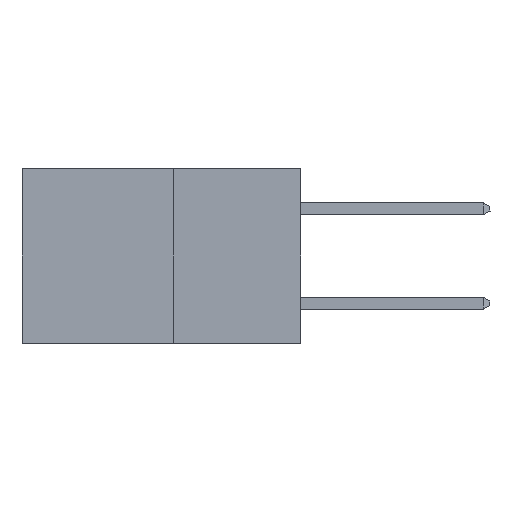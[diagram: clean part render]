
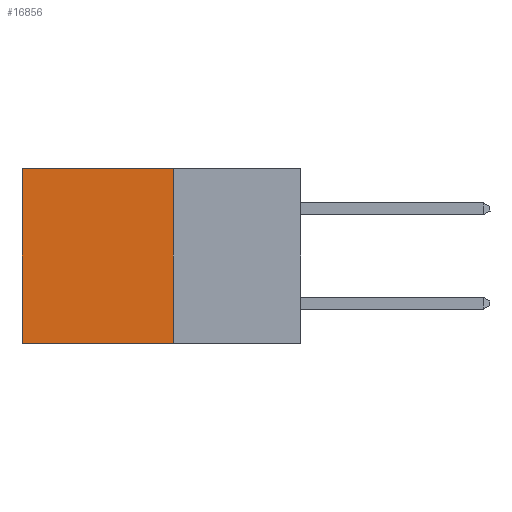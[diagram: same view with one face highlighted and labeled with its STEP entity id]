
A CAD part, left-side view. The second image highlights one B-rep face of the part: STEP entity #16856.
In plain terms, the highlighted planar face has unit normal (-1, 0, 0).
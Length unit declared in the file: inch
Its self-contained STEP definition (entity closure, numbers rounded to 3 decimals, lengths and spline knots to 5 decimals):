
#135 = DIRECTION ( 'NONE',  ( 1., 0., 0. ) ) ;
#337 = DIRECTION ( 'NONE',  ( 0., 0., -1. ) ) ;
#3577 = ORIENTED_EDGE ( 'NONE', *, *, #6771, .T. ) ;
#4001 = VECTOR ( 'NONE', #11447, 39.37008 ) ;
#5173 = CARTESIAN_POINT ( 'NONE',  ( 0.277, 0.59, -0.37 ) ) ;
#6661 = PLANE ( 'NONE',  #17743 ) ;
#6771 = EDGE_CURVE ( 'NONE', #9305, #20219, #13177, .T. ) ;
#7927 = EDGE_LOOP ( 'NONE', ( #3577, #9611, #12862, #16972 ) ) ;
#8671 = VECTOR ( 'NONE', #20311, 39.37008 ) ;
#9046 = VECTOR ( 'NONE', #18298, 39.37008 ) ;
#9305 = VERTEX_POINT ( 'NONE', #15553 ) ;
#9477 = CARTESIAN_POINT ( 'NONE',  ( 0.277, 0.27, 0. ) ) ;
#9611 = ORIENTED_EDGE ( 'NONE', *, *, #10947, .F. ) ;
#9889 = CARTESIAN_POINT ( 'NONE',  ( 0.277, 0.27, -0.37 ) ) ;
#10947 = EDGE_CURVE ( 'NONE', #12393, #20219, #12300, .T. ) ;
#11379 = EDGE_CURVE ( 'NONE', #12591, #9305, #17414, .T. ) ;
#11447 = DIRECTION ( 'NONE',  ( 0., 1., 0. ) ) ;
#12040 = CARTESIAN_POINT ( 'NONE',  ( 0.277, 0.59, -0.37 ) ) ;
#12300 = LINE ( 'NONE', #9889, #4001 ) ;
#12393 = VERTEX_POINT ( 'NONE', #12434 ) ;
#12434 = CARTESIAN_POINT ( 'NONE',  ( 0.277, 0.27, -0.37 ) ) ;
#12591 = VERTEX_POINT ( 'NONE', #12832 ) ;
#12832 = CARTESIAN_POINT ( 'NONE',  ( 0.277, 0.27, 0. ) ) ;
#12862 = ORIENTED_EDGE ( 'NONE', *, *, #15472, .F. ) ;
#13177 = LINE ( 'NONE', #12040, #9046 ) ;
#14439 = CARTESIAN_POINT ( 'NONE',  ( 0.277, 0.27, -0.37 ) ) ;
#14597 = VECTOR ( 'NONE', #337, 39.37008 ) ;
#15472 = EDGE_CURVE ( 'NONE', #12591, #12393, #18253, .T. ) ;
#15553 = CARTESIAN_POINT ( 'NONE',  ( 0.277, 0.59, 0. ) ) ;
#16856 = ADVANCED_FACE ( 'NONE', ( #18196 ), #6661, .F. ) ;
#16972 = ORIENTED_EDGE ( 'NONE', *, *, #11379, .T. ) ;
#17414 = LINE ( 'NONE', #9477, #8671 ) ;
#17588 = DIRECTION ( 'NONE',  ( 0., 0., -1. ) ) ;
#17703 = CARTESIAN_POINT ( 'NONE',  ( 0.277, 0.27, -0.37 ) ) ;
#17743 = AXIS2_PLACEMENT_3D ( 'NONE', #14439, #135, #17588 ) ;
#18196 = FACE_OUTER_BOUND ( 'NONE', #7927, .T. ) ;
#18253 = LINE ( 'NONE', #17703, #14597 ) ;
#18298 = DIRECTION ( 'NONE',  ( 0., 0., -1. ) ) ;
#20219 = VERTEX_POINT ( 'NONE', #5173 ) ;
#20311 = DIRECTION ( 'NONE',  ( 0., 1., 0. ) ) ;
